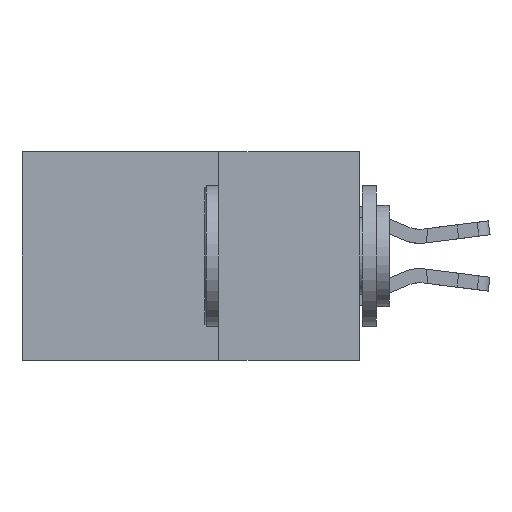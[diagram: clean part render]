
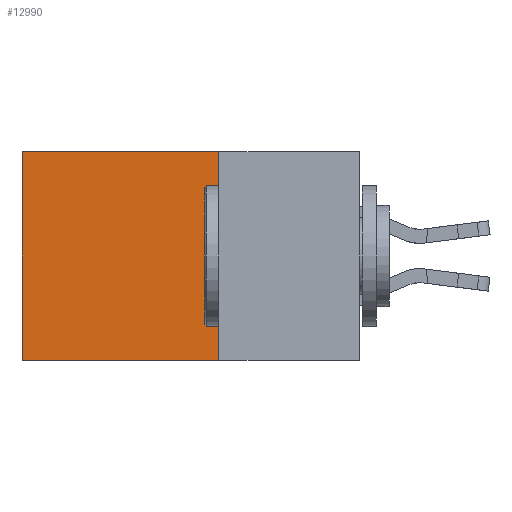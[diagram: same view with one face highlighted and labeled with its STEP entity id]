
A CAD part, left-side view. The second image highlights one B-rep face of the part: STEP entity #12990.
In plain terms, the highlighted planar face has unit normal (-1, 0, 0).
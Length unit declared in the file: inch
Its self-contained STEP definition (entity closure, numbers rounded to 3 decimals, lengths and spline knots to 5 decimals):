
#875 = LINE ( 'NONE', #31601, #7271 ) ;
#2042 = ORIENTED_EDGE ( 'NONE', *, *, #11735, .T. ) ;
#2832 = DIRECTION ( 'NONE',  ( 0., 0., -1. ) ) ;
#3101 = EDGE_CURVE ( 'NONE', #3935, #4742, #20573, .T. ) ;
#3935 = VERTEX_POINT ( 'NONE', #24840 ) ;
#3946 = LINE ( 'NONE', #29408, #25362 ) ;
#4742 = VERTEX_POINT ( 'NONE', #32454 ) ;
#6239 = VECTOR ( 'NONE', #8155, 39.37008 ) ;
#7271 = VECTOR ( 'NONE', #26329, 39.37008 ) ;
#8115 = VECTOR ( 'NONE', #2832, 39.37008 ) ;
#8119 = FACE_OUTER_BOUND ( 'NONE', #21615, .T. ) ;
#8155 = DIRECTION ( 'NONE',  ( 0., 1., 0. ) ) ;
#10786 = DIRECTION ( 'NONE',  ( 0., 0., -1. ) ) ;
#11735 = EDGE_CURVE ( 'NONE', #4742, #24073, #3946, .T. ) ;
#12166 = VERTEX_POINT ( 'NONE', #23061 ) ;
#12919 = DIRECTION ( 'NONE',  ( 1., 0., 0. ) ) ;
#12990 = ADVANCED_FACE ( 'NONE', ( #8119 ), #26113, .F. ) ;
#13027 = EDGE_CURVE ( 'NONE', #12166, #24073, #875, .T. ) ;
#13578 = CARTESIAN_POINT ( 'NONE',  ( 0.2875, 0.25, 0. ) ) ;
#15281 = LINE ( 'NONE', #13578, #8115 ) ;
#17697 = EDGE_CURVE ( 'NONE', #3935, #12166, #15281, .T. ) ;
#18906 = ORIENTED_EDGE ( 'NONE', *, *, #13027, .F. ) ;
#20573 = LINE ( 'NONE', #24216, #6239 ) ;
#21615 = EDGE_LOOP ( 'NONE', ( #2042, #18906, #25063, #24962 ) ) ;
#23061 = CARTESIAN_POINT ( 'NONE',  ( 0.2875, 0.25, -0.37 ) ) ;
#24073 = VERTEX_POINT ( 'NONE', #25761 ) ;
#24216 = CARTESIAN_POINT ( 'NONE',  ( 0.2875, 0.25, 0. ) ) ;
#24840 = CARTESIAN_POINT ( 'NONE',  ( 0.2875, 0.25, 0. ) ) ;
#24962 = ORIENTED_EDGE ( 'NONE', *, *, #3101, .T. ) ;
#25063 = ORIENTED_EDGE ( 'NONE', *, *, #17697, .F. ) ;
#25362 = VECTOR ( 'NONE', #10786, 39.37008 ) ;
#25761 = CARTESIAN_POINT ( 'NONE',  ( 0.2875, 0.6, -0.37 ) ) ;
#26113 = PLANE ( 'NONE',  #26988 ) ;
#26329 = DIRECTION ( 'NONE',  ( 0., 1., 0. ) ) ;
#26988 = AXIS2_PLACEMENT_3D ( 'NONE', #28865, #12919, #31481 ) ;
#28865 = CARTESIAN_POINT ( 'NONE',  ( 0.2875, 0.25, 0. ) ) ;
#29408 = CARTESIAN_POINT ( 'NONE',  ( 0.2875, 0.6, 0. ) ) ;
#31481 = DIRECTION ( 'NONE',  ( 0., 0., -1. ) ) ;
#31601 = CARTESIAN_POINT ( 'NONE',  ( 0.2875, 0.25, -0.37 ) ) ;
#32454 = CARTESIAN_POINT ( 'NONE',  ( 0.2875, 0.6, 0. ) ) ;
